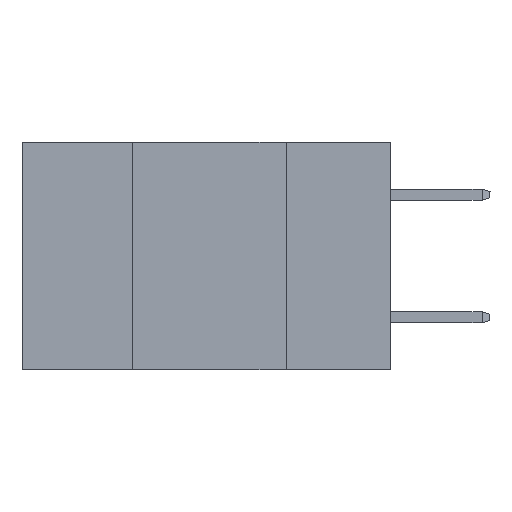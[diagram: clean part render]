
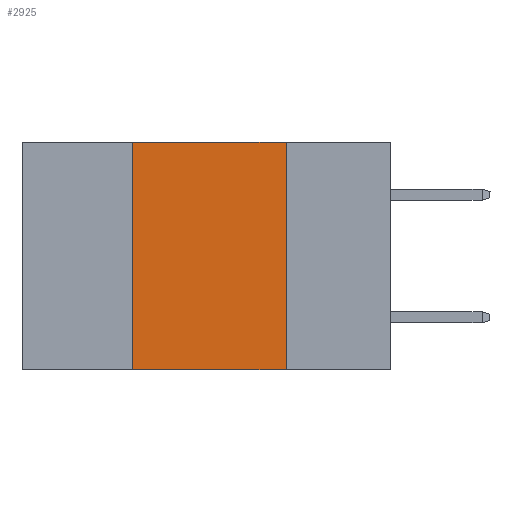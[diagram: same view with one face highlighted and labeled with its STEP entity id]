
A CAD part, left-side view. The second image highlights one B-rep face of the part: STEP entity #2925.
In plain terms, the highlighted planar face has unit normal (-1, 0, 0).
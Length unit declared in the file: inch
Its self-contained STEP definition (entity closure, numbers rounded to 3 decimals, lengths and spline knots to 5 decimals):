
#121 = DIRECTION ( 'NONE',  ( 0., 0., -1. ) ) ;
#506 = VERTEX_POINT ( 'NONE', #3199 ) ;
#1533 = DIRECTION ( 'NONE',  ( 1., 0., 0. ) ) ;
#1572 = ORIENTED_EDGE ( 'NONE', *, *, #11270, .F. ) ;
#1864 = VECTOR ( 'NONE', #5838, 39.37008 ) ;
#1950 = ORIENTED_EDGE ( 'NONE', *, *, #6567, .F. ) ;
#2049 = ORIENTED_EDGE ( 'NONE', *, *, #4665, .F. ) ;
#2088 = PLANE ( 'NONE',  #6743 ) ;
#2111 = ORIENTED_EDGE ( 'NONE', *, *, #12183, .T. ) ;
#2183 = LINE ( 'NONE', #8826, #10236 ) ;
#2604 = EDGE_LOOP ( 'NONE', ( #1572, #1950, #2049, #2111 ) ) ;
#2688 = DIRECTION ( 'NONE',  ( 0., 0., 1. ) ) ;
#2925 = ADVANCED_FACE ( 'NONE', ( #11037 ), #2088, .F. ) ;
#3199 = CARTESIAN_POINT ( 'NONE',  ( 0., 0.17, -0.37 ) ) ;
#3394 = CARTESIAN_POINT ( 'NONE',  ( 0., 0.6, -0.37 ) ) ;
#4665 = EDGE_CURVE ( 'NONE', #10957, #6360, #2183, .T. ) ;
#4906 = LINE ( 'NONE', #3394, #12142 ) ;
#5409 = VECTOR ( 'NONE', #11584, 39.37008 ) ;
#5838 = DIRECTION ( 'NONE',  ( 0., -1., 0. ) ) ;
#6360 = VERTEX_POINT ( 'NONE', #9583 ) ;
#6567 = EDGE_CURVE ( 'NONE', #6360, #12426, #12513, .T. ) ;
#6604 = DIRECTION ( 'NONE',  ( 0., -1., 0. ) ) ;
#6691 = CARTESIAN_POINT ( 'NONE',  ( 0., 0.6, 0. ) ) ;
#6743 = AXIS2_PLACEMENT_3D ( 'NONE', #6691, #1533, #121 ) ;
#7713 = CARTESIAN_POINT ( 'NONE',  ( 0., 0.17, 0. ) ) ;
#7847 = CARTESIAN_POINT ( 'NONE',  ( 0., 0.17, 0. ) ) ;
#8826 = CARTESIAN_POINT ( 'NONE',  ( 0., 0.42, 0. ) ) ;
#9583 = CARTESIAN_POINT ( 'NONE',  ( 0., 0.42, 0. ) ) ;
#9742 = CARTESIAN_POINT ( 'NONE',  ( 0., 0.6, 0. ) ) ;
#10236 = VECTOR ( 'NONE', #2688, 39.37008 ) ;
#10617 = LINE ( 'NONE', #7713, #5409 ) ;
#10957 = VERTEX_POINT ( 'NONE', #12244 ) ;
#11037 = FACE_OUTER_BOUND ( 'NONE', #2604, .T. ) ;
#11270 = EDGE_CURVE ( 'NONE', #12426, #506, #10617, .T. ) ;
#11584 = DIRECTION ( 'NONE',  ( 0., 0., -1. ) ) ;
#12142 = VECTOR ( 'NONE', #6604, 39.37008 ) ;
#12183 = EDGE_CURVE ( 'NONE', #10957, #506, #4906, .T. ) ;
#12244 = CARTESIAN_POINT ( 'NONE',  ( 0., 0.42, -0.37 ) ) ;
#12426 = VERTEX_POINT ( 'NONE', #7847 ) ;
#12513 = LINE ( 'NONE', #9742, #1864 ) ;
